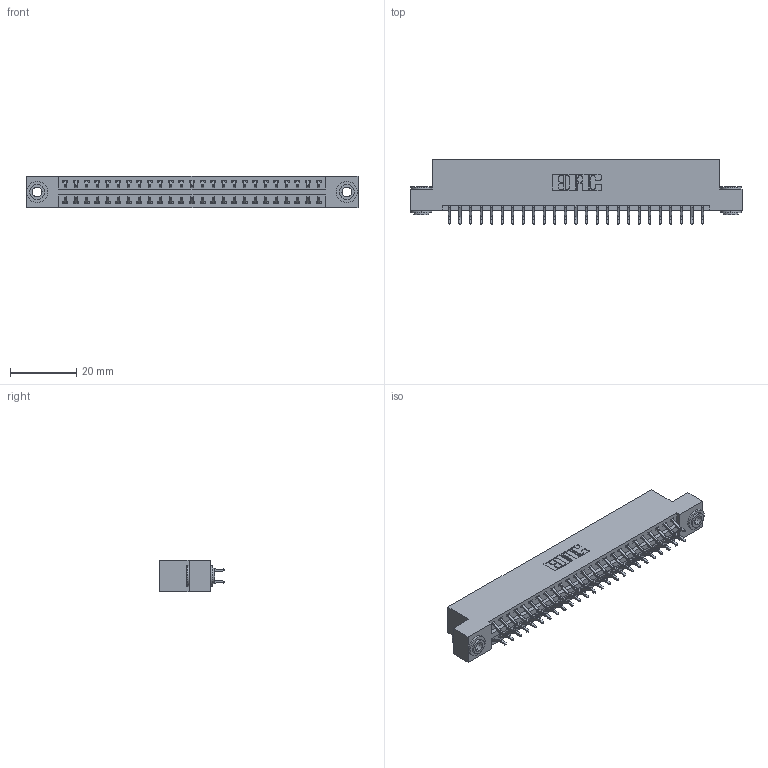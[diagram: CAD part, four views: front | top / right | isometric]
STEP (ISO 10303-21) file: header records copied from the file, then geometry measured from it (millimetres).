
FILE_DESCRIPTION (( 'STEP AP203' ), '1' );
FILE_NAME ('396-050-556-203.STEP', '2018-09-08T04:46:15', ( '' ), ( '' ), 'SwSTEP 2.0', 'SolidWorks 2016', '' );
FILE_SCHEMA (( 'CONFIG_CONTROL_DESIGN' ));
Length unit declared in the file: inch
Products named in the file (4): 346 Part_Flush Mounting Lugs - 0.156 Dia-TH; 345-292-001_556 Tail; 345-250-002_345-250-002-102; 396-050-556-203
Assembly tree (53 placements, depth 2):
  396-050-556-203
    346 Part_Flush Mounting Lugs - 0.156 Dia-TH
    345-292-001_556 Tail  x50
    345-250-002_345-250-002-102  x2
Bounding box: 99.95 x 19.57 x 9.4 mm (x, y, z)
Volume: 9631.6 mm3; surface area: 13139.9 mm2
Topology: 53 solids, 53 shells, 3060 faces, 9055 edges, 5966 vertices
Faces by surface type: plane 2036, cylinder 1016, cone 8
Entity records: 19474 total; most frequent: CARTESIAN_POINT 3223, ORIENTED_EDGE 3138, DIRECTION 2911, EDGE_CURVE 1569, VECTOR 1305, LINE 1305, VERTEX_POINT 1042, AXIS2_PLACEMENT_3D 803
